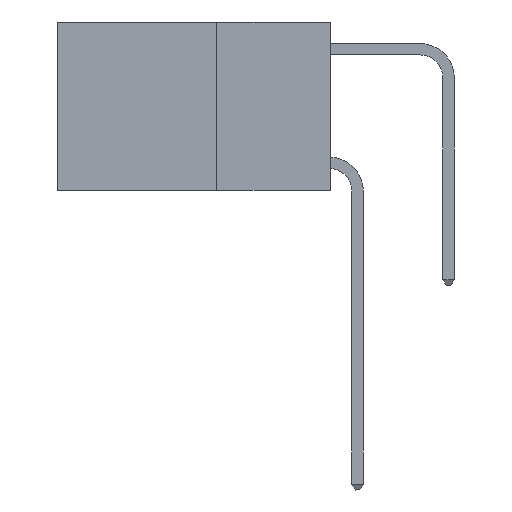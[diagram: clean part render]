
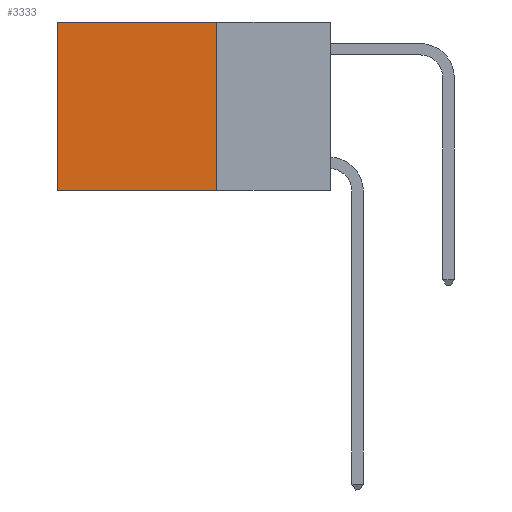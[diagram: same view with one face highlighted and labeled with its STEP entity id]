
A CAD part, left-side view. The second image highlights one B-rep face of the part: STEP entity #3333.
In plain terms, the highlighted planar face has unit normal (-1, 0, 0).
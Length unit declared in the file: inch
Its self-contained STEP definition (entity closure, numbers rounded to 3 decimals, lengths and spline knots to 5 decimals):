
#252 = VECTOR ( 'NONE', #7995, 39.37008 ) ;
#578 = DIRECTION ( 'NONE',  ( 0., 0., -1. ) ) ;
#797 = DIRECTION ( 'NONE',  ( 0., 0., -1. ) ) ;
#1094 = LINE ( 'NONE', #5671, #7653 ) ;
#1120 = VECTOR ( 'NONE', #797, 39.37008 ) ;
#1202 = EDGE_CURVE ( 'NONE', #10776, #4884, #7677, .T. ) ;
#2001 = EDGE_CURVE ( 'NONE', #8619, #10666, #3644, .T. ) ;
#2006 = ORIENTED_EDGE ( 'NONE', *, *, #7022, .T. ) ;
#2066 = FACE_OUTER_BOUND ( 'NONE', #8254, .T. ) ;
#2310 = DIRECTION ( 'NONE',  ( 0., 0., -1. ) ) ;
#2321 = CARTESIAN_POINT ( 'NONE',  ( 0.2625, 0.25, 0. ) ) ;
#2993 = CARTESIAN_POINT ( 'NONE',  ( 0.2625, 0.25, 0. ) ) ;
#3078 = CARTESIAN_POINT ( 'NONE',  ( 0.2625, 0.6, 0. ) ) ;
#3333 = ADVANCED_FACE ( 'NONE', ( #2066 ), #11192, .F. ) ;
#3344 = VECTOR ( 'NONE', #2310, 39.37008 ) ;
#3644 = LINE ( 'NONE', #6798, #3344 ) ;
#3855 = CARTESIAN_POINT ( 'NONE',  ( 0.2625, 0.6, 0. ) ) ;
#4739 = LINE ( 'NONE', #7121, #252 ) ;
#4758 = DIRECTION ( 'NONE',  ( 0., 1., 0. ) ) ;
#4884 = VERTEX_POINT ( 'NONE', #9503 ) ;
#4987 = ORIENTED_EDGE ( 'NONE', *, *, #8335, .F. ) ;
#5292 = AXIS2_PLACEMENT_3D ( 'NONE', #2321, #5971, #578 ) ;
#5671 = CARTESIAN_POINT ( 'NONE',  ( 0.2625, 0.25, 0. ) ) ;
#5971 = DIRECTION ( 'NONE',  ( 1., 0., 0. ) ) ;
#6532 = CARTESIAN_POINT ( 'NONE',  ( 0.2625, 0.25, -0.37 ) ) ;
#6798 = CARTESIAN_POINT ( 'NONE',  ( 0.2625, 0.25, 0. ) ) ;
#7022 = EDGE_CURVE ( 'NONE', #8619, #10776, #1094, .T. ) ;
#7121 = CARTESIAN_POINT ( 'NONE',  ( 0.2625, 0.25, -0.37 ) ) ;
#7653 = VECTOR ( 'NONE', #4758, 39.37008 ) ;
#7677 = LINE ( 'NONE', #3855, #1120 ) ;
#7995 = DIRECTION ( 'NONE',  ( 0., 1., 0. ) ) ;
#8254 = EDGE_LOOP ( 'NONE', ( #11164, #4987, #10486, #2006 ) ) ;
#8335 = EDGE_CURVE ( 'NONE', #10666, #4884, #4739, .T. ) ;
#8619 = VERTEX_POINT ( 'NONE', #2993 ) ;
#9503 = CARTESIAN_POINT ( 'NONE',  ( 0.2625, 0.6, -0.37 ) ) ;
#10486 = ORIENTED_EDGE ( 'NONE', *, *, #2001, .F. ) ;
#10666 = VERTEX_POINT ( 'NONE', #6532 ) ;
#10776 = VERTEX_POINT ( 'NONE', #3078 ) ;
#11164 = ORIENTED_EDGE ( 'NONE', *, *, #1202, .T. ) ;
#11192 = PLANE ( 'NONE',  #5292 ) ;
